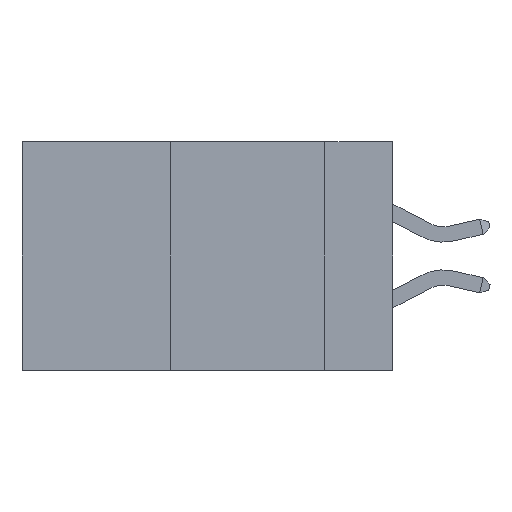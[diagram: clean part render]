
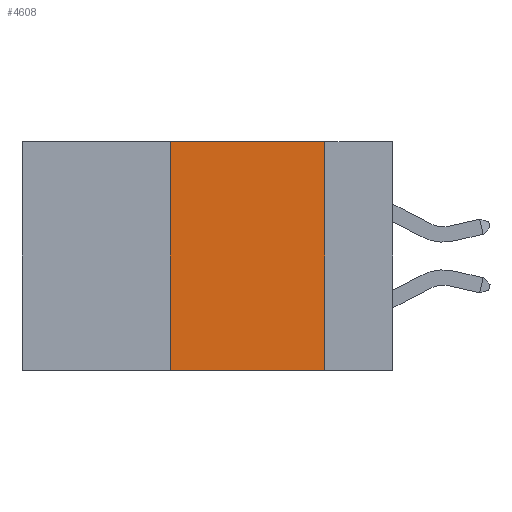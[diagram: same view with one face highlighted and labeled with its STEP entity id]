
A CAD part, left-side view. The second image highlights one B-rep face of the part: STEP entity #4608.
In plain terms, the highlighted planar face has unit normal (-1, 0, 0).
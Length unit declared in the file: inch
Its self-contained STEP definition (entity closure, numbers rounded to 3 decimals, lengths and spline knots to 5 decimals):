
#362 = EDGE_CURVE ( 'NONE', #11557, #8507, #16751, .T. ) ;
#2160 = ORIENTED_EDGE ( 'NONE', *, *, #6327, .T. ) ;
#2280 = CARTESIAN_POINT ( 'NONE',  ( 0., 0.11, -0.37 ) ) ;
#3870 = DIRECTION ( 'NONE',  ( 0., 0., -1. ) ) ;
#4600 = CARTESIAN_POINT ( 'NONE',  ( 0., 0.6, -0.37 ) ) ;
#4608 = ADVANCED_FACE ( 'NONE', ( #33386 ), #17743, .F. ) ;
#6327 = EDGE_CURVE ( 'NONE', #11557, #9107, #7261, .T. ) ;
#6564 = LINE ( 'NONE', #14303, #25692 ) ;
#6953 = ORIENTED_EDGE ( 'NONE', *, *, #10503, .F. ) ;
#7261 = LINE ( 'NONE', #4600, #24190 ) ;
#8070 = EDGE_CURVE ( 'NONE', #24997, #9107, #15472, .T. ) ;
#8507 = VERTEX_POINT ( 'NONE', #26572 ) ;
#9107 = VERTEX_POINT ( 'NONE', #2280 ) ;
#9248 = CARTESIAN_POINT ( 'NONE',  ( 0., 0.6, 0. ) ) ;
#9379 = VECTOR ( 'NONE', #16073, 39.37008 ) ;
#9724 = EDGE_LOOP ( 'NONE', ( #13055, #6953, #12611, #2160 ) ) ;
#10503 = EDGE_CURVE ( 'NONE', #8507, #24997, #6564, .T. ) ;
#11221 = CARTESIAN_POINT ( 'NONE',  ( 0., 0.11, 0. ) ) ;
#11557 = VERTEX_POINT ( 'NONE', #13847 ) ;
#11759 = DIRECTION ( 'NONE',  ( 0., -1., 0. ) ) ;
#12611 = ORIENTED_EDGE ( 'NONE', *, *, #362, .F. ) ;
#12867 = VECTOR ( 'NONE', #26872, 39.37008 ) ;
#13038 = CARTESIAN_POINT ( 'NONE',  ( 0., 0.11, 0. ) ) ;
#13055 = ORIENTED_EDGE ( 'NONE', *, *, #8070, .F. ) ;
#13396 = CARTESIAN_POINT ( 'NONE',  ( 0., 0.36, 0. ) ) ;
#13847 = CARTESIAN_POINT ( 'NONE',  ( 0., 0.36, -0.37 ) ) ;
#14303 = CARTESIAN_POINT ( 'NONE',  ( 0., 0.6, 0. ) ) ;
#14419 = DIRECTION ( 'NONE',  ( 1., 0., 0. ) ) ;
#15472 = LINE ( 'NONE', #13038, #12867 ) ;
#16073 = DIRECTION ( 'NONE',  ( 0., 0., 1. ) ) ;
#16751 = LINE ( 'NONE', #13396, #9379 ) ;
#17743 = PLANE ( 'NONE',  #30159 ) ;
#24190 = VECTOR ( 'NONE', #26779, 39.37008 ) ;
#24997 = VERTEX_POINT ( 'NONE', #11221 ) ;
#25692 = VECTOR ( 'NONE', #11759, 39.37008 ) ;
#26572 = CARTESIAN_POINT ( 'NONE',  ( 0., 0.36, 0. ) ) ;
#26779 = DIRECTION ( 'NONE',  ( 0., -1., 0. ) ) ;
#26872 = DIRECTION ( 'NONE',  ( 0., 0., -1. ) ) ;
#30159 = AXIS2_PLACEMENT_3D ( 'NONE', #9248, #14419, #3870 ) ;
#33386 = FACE_OUTER_BOUND ( 'NONE', #9724, .T. ) ;
